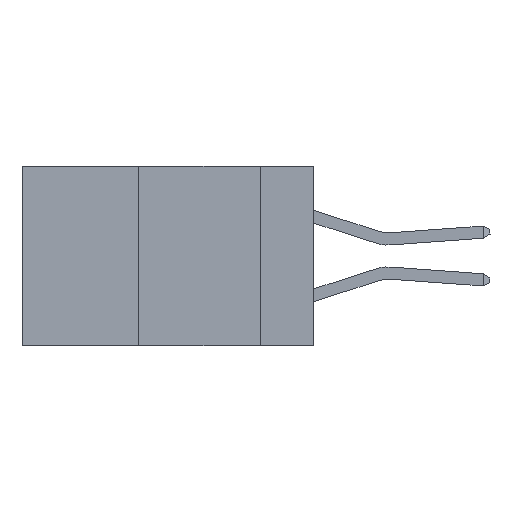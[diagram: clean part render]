
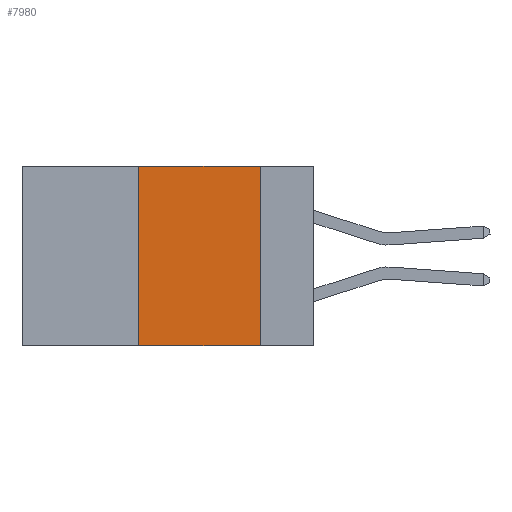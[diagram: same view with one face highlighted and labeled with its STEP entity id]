
A CAD part, left-side view. The second image highlights one B-rep face of the part: STEP entity #7980.
In plain terms, the highlighted planar face has unit normal (-1, 0, 0).
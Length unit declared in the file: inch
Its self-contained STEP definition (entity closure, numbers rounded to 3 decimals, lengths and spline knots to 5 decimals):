
#109 = EDGE_LOOP ( 'NONE', ( #7862, #6737, #6529, #5523 ) ) ;
#505 = AXIS2_PLACEMENT_3D ( 'NONE', #5732, #9096, #10543 ) ;
#702 = DIRECTION ( 'NONE',  ( 0., 0., -1. ) ) ;
#737 = VERTEX_POINT ( 'NONE', #5118 ) ;
#870 = VECTOR ( 'NONE', #702, 39.37008 ) ;
#1495 = CARTESIAN_POINT ( 'NONE',  ( 0., 0.11, -0.37 ) ) ;
#2418 = FACE_OUTER_BOUND ( 'NONE', #109, .T. ) ;
#2435 = LINE ( 'NONE', #9057, #9218 ) ;
#2782 = CARTESIAN_POINT ( 'NONE',  ( 0., 0.6, -0.37 ) ) ;
#2783 = EDGE_CURVE ( 'NONE', #6220, #3868, #5942, .T. ) ;
#3078 = CARTESIAN_POINT ( 'NONE',  ( 0., 0.36, -0.37 ) ) ;
#3089 = VECTOR ( 'NONE', #3534, 39.37008 ) ;
#3534 = DIRECTION ( 'NONE',  ( 0., -1., 0. ) ) ;
#3609 = CARTESIAN_POINT ( 'NONE',  ( 0., 0.11, 0. ) ) ;
#3868 = VERTEX_POINT ( 'NONE', #1495 ) ;
#4260 = DIRECTION ( 'NONE',  ( 0., -1., 0. ) ) ;
#4616 = EDGE_CURVE ( 'NONE', #6220, #737, #2435, .T. ) ;
#4713 = PLANE ( 'NONE',  #505 ) ;
#4818 = VERTEX_POINT ( 'NONE', #3609 ) ;
#5118 = CARTESIAN_POINT ( 'NONE',  ( 0., 0.36, 0. ) ) ;
#5523 = ORIENTED_EDGE ( 'NONE', *, *, #2783, .T. ) ;
#5732 = CARTESIAN_POINT ( 'NONE',  ( 0., 0.6, 0. ) ) ;
#5942 = LINE ( 'NONE', #2782, #3089 ) ;
#6220 = VERTEX_POINT ( 'NONE', #3078 ) ;
#6529 = ORIENTED_EDGE ( 'NONE', *, *, #4616, .F. ) ;
#6713 = LINE ( 'NONE', #8418, #9258 ) ;
#6737 = ORIENTED_EDGE ( 'NONE', *, *, #8084, .F. ) ;
#7307 = CARTESIAN_POINT ( 'NONE',  ( 0., 0.11, 0. ) ) ;
#7862 = ORIENTED_EDGE ( 'NONE', *, *, #8404, .F. ) ;
#7980 = ADVANCED_FACE ( 'NONE', ( #2418 ), #4713, .F. ) ;
#8084 = EDGE_CURVE ( 'NONE', #737, #4818, #6713, .T. ) ;
#8176 = DIRECTION ( 'NONE',  ( 0., 0., 1. ) ) ;
#8404 = EDGE_CURVE ( 'NONE', #4818, #3868, #8861, .T. ) ;
#8418 = CARTESIAN_POINT ( 'NONE',  ( 0., 0.6, 0. ) ) ;
#8861 = LINE ( 'NONE', #7307, #870 ) ;
#9057 = CARTESIAN_POINT ( 'NONE',  ( 0., 0.36, 0. ) ) ;
#9096 = DIRECTION ( 'NONE',  ( 1., 0., 0. ) ) ;
#9218 = VECTOR ( 'NONE', #8176, 39.37008 ) ;
#9258 = VECTOR ( 'NONE', #4260, 39.37008 ) ;
#10543 = DIRECTION ( 'NONE',  ( 0., 0., -1. ) ) ;
